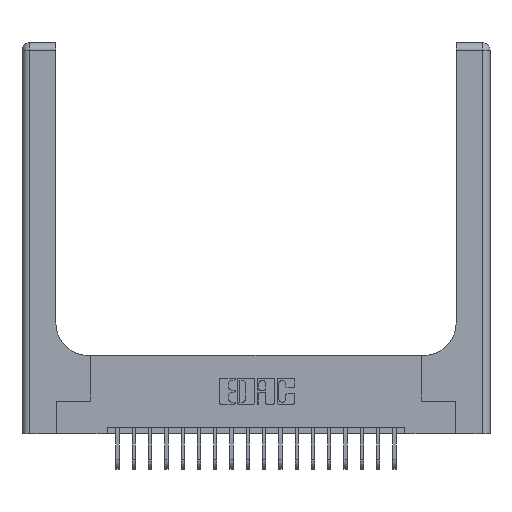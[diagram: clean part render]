
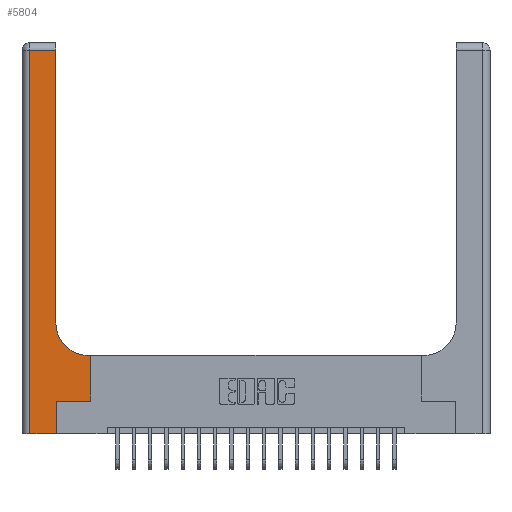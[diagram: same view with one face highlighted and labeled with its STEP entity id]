
A CAD part, top view. The second image highlights one B-rep face of the part: STEP entity #5804.
In plain terms, the highlighted planar face has unit normal (0, 0, 1).
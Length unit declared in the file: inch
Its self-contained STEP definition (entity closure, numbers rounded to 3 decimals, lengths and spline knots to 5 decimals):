
#798 = VECTOR ( 'NONE', #21344, 39.37008 ) ;
#909 = VERTEX_POINT ( 'NONE', #13241 ) ;
#1042 = EDGE_CURVE ( 'NONE', #10435, #1152, #20441, .T. ) ;
#1149 = ORIENTED_EDGE ( 'NONE', *, *, #19432, .T. ) ;
#1152 = VERTEX_POINT ( 'NONE', #3967 ) ;
#1205 = VECTOR ( 'NONE', #3619, 39.37008 ) ;
#1934 = LINE ( 'NONE', #15959, #3884 ) ;
#2094 = VECTOR ( 'NONE', #12195, 39.37008 ) ;
#2354 = LINE ( 'NONE', #5296, #2094 ) ;
#3299 = EDGE_CURVE ( 'NONE', #20345, #5258, #1934, .T. ) ;
#3619 = DIRECTION ( 'NONE',  ( -1., 0., 0. ) ) ;
#3628 = DIRECTION ( 'NONE',  ( 0., 1., 0. ) ) ;
#3653 = DIRECTION ( 'NONE',  ( 1., 0., 0. ) ) ;
#3884 = VECTOR ( 'NONE', #15843, 39.37008 ) ;
#3967 = CARTESIAN_POINT ( 'NONE',  ( 0.26, 0.85, 0.37 ) ) ;
#4543 = DIRECTION ( 'NONE',  ( -1., 0., 0. ) ) ;
#5258 = VERTEX_POINT ( 'NONE', #11667 ) ;
#5296 = CARTESIAN_POINT ( 'NONE',  ( 0., 0., 0.37 ) ) ;
#5437 = VECTOR ( 'NONE', #17940, 39.37008 ) ;
#5804 = ADVANCED_FACE ( 'NONE', ( #21961 ), #11898, .F. ) ;
#6038 = ORIENTED_EDGE ( 'NONE', *, *, #13189, .T. ) ;
#6092 = EDGE_CURVE ( 'NONE', #909, #10435, #15104, .T. ) ;
#6373 = ORIENTED_EDGE ( 'NONE', *, *, #13536, .T. ) ;
#6801 = CARTESIAN_POINT ( 'NONE',  ( 0.51, 0.85, 0.37 ) ) ;
#6900 = DIRECTION ( 'NONE',  ( 0., 0., -1. ) ) ;
#7360 = CARTESIAN_POINT ( 'NONE',  ( 0.265, 0.25, 0.37 ) ) ;
#7501 = VERTEX_POINT ( 'NONE', #19981 ) ;
#8324 = VECTOR ( 'NONE', #3628, 39.37008 ) ;
#8394 = CARTESIAN_POINT ( 'NONE',  ( 0., 3., 0.37 ) ) ;
#8757 = CARTESIAN_POINT ( 'NONE',  ( 0.528, 0.25, 0.37 ) ) ;
#8804 = EDGE_CURVE ( 'NONE', #7501, #20345, #2354, .T. ) ;
#8919 = AXIS2_PLACEMENT_3D ( 'NONE', #8394, #22192, #4543 ) ;
#9126 = LINE ( 'NONE', #18167, #798 ) ;
#9631 = ORIENTED_EDGE ( 'NONE', *, *, #15698, .T. ) ;
#9780 = VECTOR ( 'NONE', #3653, 39.37008 ) ;
#10056 = ORIENTED_EDGE ( 'NONE', *, *, #14037, .T. ) ;
#10136 = CARTESIAN_POINT ( 'NONE',  ( 0.26, 2.94, 0.37 ) ) ;
#10435 = VERTEX_POINT ( 'NONE', #17238 ) ;
#10525 = AXIS2_PLACEMENT_3D ( 'NONE', #6801, #6900, #11549 ) ;
#10746 = LINE ( 'NONE', #19071, #8324 ) ;
#11049 = LINE ( 'NONE', #21221, #5437 ) ;
#11549 = DIRECTION ( 'NONE',  ( 1., 0., 0. ) ) ;
#11599 = ORIENTED_EDGE ( 'NONE', *, *, #3299, .T. ) ;
#11667 = CARTESIAN_POINT ( 'NONE',  ( 0.265, 0.25, 0.37 ) ) ;
#11898 = PLANE ( 'NONE',  #8919 ) ;
#12195 = DIRECTION ( 'NONE',  ( 1., 0., 0. ) ) ;
#12280 = ORIENTED_EDGE ( 'NONE', *, *, #1042, .T. ) ;
#12912 = EDGE_LOOP ( 'NONE', ( #9631, #1149, #10056, #16674, #11599, #6038, #6373, #18512, #12280 ) ) ;
#13082 = VERTEX_POINT ( 'NONE', #10136 ) ;
#13189 = EDGE_CURVE ( 'NONE', #5258, #21773, #19569, .T. ) ;
#13241 = CARTESIAN_POINT ( 'NONE',  ( 0.528, 0.6, 0.37 ) ) ;
#13515 = CARTESIAN_POINT ( 'NONE',  ( 0.265, 0., 0.37 ) ) ;
#13536 = EDGE_CURVE ( 'NONE', #21773, #909, #10746, .T. ) ;
#14037 = EDGE_CURVE ( 'NONE', #17373, #7501, #11049, .T. ) ;
#15104 = LINE ( 'NONE', #20297, #16876 ) ;
#15698 = EDGE_CURVE ( 'NONE', #1152, #13082, #9126, .T. ) ;
#15843 = DIRECTION ( 'NONE',  ( 0., 1., 0. ) ) ;
#15959 = CARTESIAN_POINT ( 'NONE',  ( 0.265, 0., 0.37 ) ) ;
#16674 = ORIENTED_EDGE ( 'NONE', *, *, #8804, .T. ) ;
#16876 = VECTOR ( 'NONE', #18141, 39.37008 ) ;
#17238 = CARTESIAN_POINT ( 'NONE',  ( 0.51, 0.6, 0.37 ) ) ;
#17373 = VERTEX_POINT ( 'NONE', #18851 ) ;
#17940 = DIRECTION ( 'NONE',  ( 0., -1., 0. ) ) ;
#18141 = DIRECTION ( 'NONE',  ( -1., 0., 0. ) ) ;
#18167 = CARTESIAN_POINT ( 'NONE',  ( 0.26, 3., 0.37 ) ) ;
#18512 = ORIENTED_EDGE ( 'NONE', *, *, #6092, .T. ) ;
#18851 = CARTESIAN_POINT ( 'NONE',  ( 0.06, 2.94, 0.37 ) ) ;
#19071 = CARTESIAN_POINT ( 'NONE',  ( 0.528, 0.25, 0.37 ) ) ;
#19416 = LINE ( 'NONE', #19525, #1205 ) ;
#19432 = EDGE_CURVE ( 'NONE', #13082, #17373, #19416, .T. ) ;
#19525 = CARTESIAN_POINT ( 'NONE',  ( 0., 2.94, 0.37 ) ) ;
#19569 = LINE ( 'NONE', #7360, #9780 ) ;
#19981 = CARTESIAN_POINT ( 'NONE',  ( 0.06, 0., 0.37 ) ) ;
#20297 = CARTESIAN_POINT ( 'NONE',  ( 0.26, 0.6, 0.37 ) ) ;
#20345 = VERTEX_POINT ( 'NONE', #13515 ) ;
#20441 = CIRCLE ( 'NONE', #10525, 0.25 ) ;
#21221 = CARTESIAN_POINT ( 'NONE',  ( 0.06, 3., 0.37 ) ) ;
#21344 = DIRECTION ( 'NONE',  ( 0., 1., 0. ) ) ;
#21773 = VERTEX_POINT ( 'NONE', #8757 ) ;
#21961 = FACE_OUTER_BOUND ( 'NONE', #12912, .T. ) ;
#22192 = DIRECTION ( 'NONE',  ( 0., 0., -1. ) ) ;
